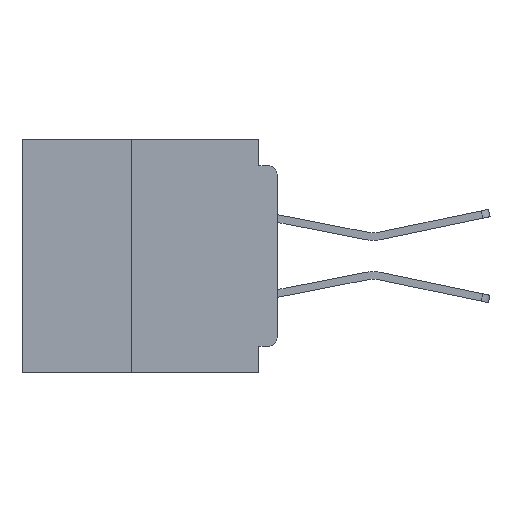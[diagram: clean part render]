
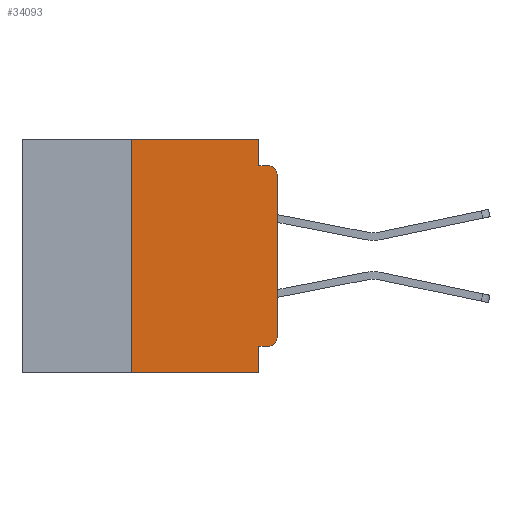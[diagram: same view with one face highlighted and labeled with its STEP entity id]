
A CAD part, left-side view. The second image highlights one B-rep face of the part: STEP entity #34093.
In plain terms, the highlighted planar face has unit normal (-1, 0, 0).
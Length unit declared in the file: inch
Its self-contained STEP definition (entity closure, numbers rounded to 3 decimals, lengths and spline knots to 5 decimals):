
#301 = CARTESIAN_POINT ( 'NONE',  ( 0., 0.437, 0. ) ) ;
#578 = EDGE_CURVE ( 'NONE', #30270, #25019, #24374, .T. ) ;
#1362 = EDGE_CURVE ( 'NONE', #44994, #8037, #17791, .T. ) ;
#3659 = CARTESIAN_POINT ( 'NONE',  ( 0., 0.031, -0.045 ) ) ;
#3693 = CARTESIAN_POINT ( 'NONE',  ( 0., 0.25, -0.4 ) ) ;
#4317 = CARTESIAN_POINT ( 'NONE',  ( 0., 0.015, -0.06 ) ) ;
#5794 = AXIS2_PLACEMENT_3D ( 'NONE', #301, #19275, #45634 ) ;
#6305 = AXIS2_PLACEMENT_3D ( 'NONE', #4317, #30686, #8091 ) ;
#7229 = LINE ( 'NONE', #36930, #26130 ) ;
#7628 = DIRECTION ( 'NONE',  ( 0., -1., 0. ) ) ;
#7691 = VECTOR ( 'NONE', #30550, 39.37008 ) ;
#8037 = VERTEX_POINT ( 'NONE', #31491 ) ;
#8091 = DIRECTION ( 'NONE',  ( 0., 0., -1. ) ) ;
#8639 = DIRECTION ( 'NONE',  ( 0., 1., 0. ) ) ;
#8854 = CARTESIAN_POINT ( 'NONE',  ( 0., 0.437, 0. ) ) ;
#9461 = VERTEX_POINT ( 'NONE', #21530 ) ;
#10641 = EDGE_CURVE ( 'NONE', #21918, #25019, #27790, .T. ) ;
#10883 = VECTOR ( 'NONE', #16834, 39.37008 ) ;
#12059 = EDGE_CURVE ( 'NONE', #43775, #21918, #23014, .T. ) ;
#12919 = VECTOR ( 'NONE', #8639, 39.37008 ) ;
#13470 = CARTESIAN_POINT ( 'NONE',  ( 0., 0.015, -0.34 ) ) ;
#13610 = CARTESIAN_POINT ( 'NONE',  ( 0., 0.25, 0. ) ) ;
#16600 = VECTOR ( 'NONE', #7628, 39.37008 ) ;
#16683 = EDGE_CURVE ( 'NONE', #8037, #25444, #7229, .T. ) ;
#16834 = DIRECTION ( 'NONE',  ( 0., -1., 0. ) ) ;
#16992 = CARTESIAN_POINT ( 'NONE',  ( 0., 0., -0.045 ) ) ;
#17333 = DIRECTION ( 'NONE',  ( 0., 0., -1. ) ) ;
#17791 = LINE ( 'NONE', #8854, #16600 ) ;
#18489 = EDGE_CURVE ( 'NONE', #43775, #33045, #31045, .T. ) ;
#19275 = DIRECTION ( 'NONE',  ( 1., 0., 0. ) ) ;
#19359 = EDGE_CURVE ( 'NONE', #25444, #34838, #41008, .T. ) ;
#19865 = CARTESIAN_POINT ( 'NONE',  ( 0., 0.015, -0.045 ) ) ;
#21530 = CARTESIAN_POINT ( 'NONE',  ( 0., 0., -0.06 ) ) ;
#21918 = VERTEX_POINT ( 'NONE', #30055 ) ;
#21957 = DIRECTION ( 'NONE',  ( 0., 0., -1. ) ) ;
#22133 = CARTESIAN_POINT ( 'NONE',  ( 0., 0., 0. ) ) ;
#22257 = CARTESIAN_POINT ( 'NONE',  ( 0., 0., -0.34 ) ) ;
#23014 = LINE ( 'NONE', #31249, #12919 ) ;
#24374 = LINE ( 'NONE', #43133, #43231 ) ;
#25019 = VERTEX_POINT ( 'NONE', #31238 ) ;
#25444 = VERTEX_POINT ( 'NONE', #3659 ) ;
#26130 = VECTOR ( 'NONE', #21957, 39.37008 ) ;
#26466 = DIRECTION ( 'NONE',  ( 0., 0., 1. ) ) ;
#26524 = AXIS2_PLACEMENT_3D ( 'NONE', #13470, #39904, #17333 ) ;
#26791 = CARTESIAN_POINT ( 'NONE',  ( 0., 0.031, -0.4 ) ) ;
#27790 = LINE ( 'NONE', #26791, #7691 ) ;
#30055 = CARTESIAN_POINT ( 'NONE',  ( 0., 0.031, -0.355 ) ) ;
#30270 = VERTEX_POINT ( 'NONE', #43487 ) ;
#30550 = DIRECTION ( 'NONE',  ( 0., 0., -1. ) ) ;
#30686 = DIRECTION ( 'NONE',  ( -1., 0., 0. ) ) ;
#31045 = CIRCLE ( 'NONE', #26524, 0.015 ) ;
#31238 = CARTESIAN_POINT ( 'NONE',  ( 0., 0.031, -0.4 ) ) ;
#31249 = CARTESIAN_POINT ( 'NONE',  ( 0., 0., -0.355 ) ) ;
#31491 = CARTESIAN_POINT ( 'NONE',  ( 0., 0.031, 0. ) ) ;
#31827 = EDGE_CURVE ( 'NONE', #30270, #44994, #47453, .T. ) ;
#33045 = VERTEX_POINT ( 'NONE', #22257 ) ;
#34093 = ADVANCED_FACE ( 'NONE', ( #45531 ), #34227, .F. ) ;
#34227 = PLANE ( 'NONE',  #5794 ) ;
#34838 = VERTEX_POINT ( 'NONE', #19865 ) ;
#36930 = CARTESIAN_POINT ( 'NONE',  ( 0., 0.031, 0. ) ) ;
#37123 = DIRECTION ( 'NONE',  ( 0., 0., 1. ) ) ;
#39496 = LINE ( 'NONE', #22133, #48287 ) ;
#39650 = EDGE_CURVE ( 'NONE', #9461, #34838, #40006, .T. ) ;
#39904 = DIRECTION ( 'NONE',  ( -1., 0., 0. ) ) ;
#40006 = CIRCLE ( 'NONE', #6305, 0.015 ) ;
#40839 = EDGE_LOOP ( 'NONE', ( #41454, #41681, #41728, #42333, #42436, #43065, #43259, #43917, #44094, #44863 ) ) ;
#41008 = LINE ( 'NONE', #16992, #10883 ) ;
#41454 = ORIENTED_EDGE ( 'NONE', *, *, #42668, .T. ) ;
#41681 = ORIENTED_EDGE ( 'NONE', *, *, #39650, .T. ) ;
#41728 = ORIENTED_EDGE ( 'NONE', *, *, #19359, .F. ) ;
#42333 = ORIENTED_EDGE ( 'NONE', *, *, #16683, .F. ) ;
#42436 = ORIENTED_EDGE ( 'NONE', *, *, #1362, .F. ) ;
#42668 = EDGE_CURVE ( 'NONE', #33045, #9461, #39496, .T. ) ;
#43031 = DIRECTION ( 'NONE',  ( 0., -1., 0. ) ) ;
#43065 = ORIENTED_EDGE ( 'NONE', *, *, #31827, .F. ) ;
#43133 = CARTESIAN_POINT ( 'NONE',  ( 0., 0.437, -0.4 ) ) ;
#43231 = VECTOR ( 'NONE', #43031, 39.37008 ) ;
#43259 = ORIENTED_EDGE ( 'NONE', *, *, #578, .T. ) ;
#43487 = CARTESIAN_POINT ( 'NONE',  ( 0., 0.25, -0.4 ) ) ;
#43775 = VERTEX_POINT ( 'NONE', #47404 ) ;
#43917 = ORIENTED_EDGE ( 'NONE', *, *, #10641, .F. ) ;
#44094 = ORIENTED_EDGE ( 'NONE', *, *, #12059, .F. ) ;
#44863 = ORIENTED_EDGE ( 'NONE', *, *, #18489, .T. ) ;
#44994 = VERTEX_POINT ( 'NONE', #13610 ) ;
#45531 = FACE_OUTER_BOUND ( 'NONE', #40839, .T. ) ;
#45634 = DIRECTION ( 'NONE',  ( 0., 0., -1. ) ) ;
#46261 = VECTOR ( 'NONE', #26466, 39.37008 ) ;
#47404 = CARTESIAN_POINT ( 'NONE',  ( 0., 0.015, -0.355 ) ) ;
#47453 = LINE ( 'NONE', #3693, #46261 ) ;
#48287 = VECTOR ( 'NONE', #37123, 39.37008 ) ;
